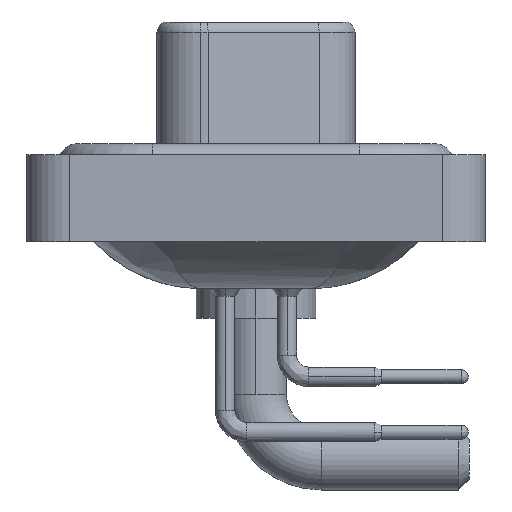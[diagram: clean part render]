
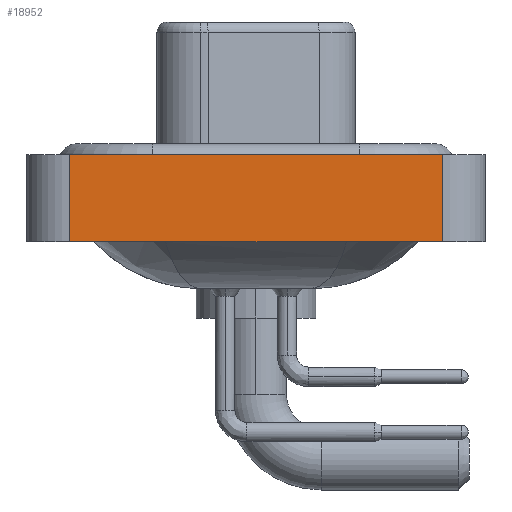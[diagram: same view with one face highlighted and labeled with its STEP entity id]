
A CAD part, left-side view. The second image highlights one B-rep face of the part: STEP entity #18952.
In plain terms, the highlighted planar face has unit normal (-1, 0, 0).
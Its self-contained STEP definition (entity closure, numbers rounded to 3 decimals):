
#564 = CARTESIAN_POINT ( 'NONE',  ( -7.25, -8.55, 0.4 ) ) ;
#1840 = AXIS2_PLACEMENT_3D ( 'NONE', #13113, #16609, #2934 ) ;
#2934 = DIRECTION ( 'NONE',  ( 0., 0., 1. ) ) ;
#3059 = ORIENTED_EDGE ( 'NONE', *, *, #8420, .T. ) ;
#3101 = EDGE_LOOP ( 'NONE', ( #10006, #10375, #14424, #3059 ) ) ;
#3458 = VERTEX_POINT ( 'NONE', #564 ) ;
#3816 = EDGE_CURVE ( 'NONE', #18432, #4788, #19182, .T. ) ;
#4437 = VECTOR ( 'NONE', #12468, 1000. ) ;
#4788 = VERTEX_POINT ( 'NONE', #21431 ) ;
#5133 = VERTEX_POINT ( 'NONE', #14258 ) ;
#5306 = EDGE_CURVE ( 'NONE', #4788, #3458, #14448, .T. ) ;
#5387 = CARTESIAN_POINT ( 'NONE',  ( -7.25, -8.55, 0.4 ) ) ;
#5415 = VECTOR ( 'NONE', #15236, 1000. ) ;
#5487 = DIRECTION ( 'NONE',  ( 0., 0., 1. ) ) ;
#7344 = CARTESIAN_POINT ( 'NONE',  ( -7.25, 8.55, -3.6 ) ) ;
#8078 = DIRECTION ( 'NONE',  ( 0., -1., 0. ) ) ;
#8420 = EDGE_CURVE ( 'NONE', #18432, #5133, #22250, .T. ) ;
#9882 = CARTESIAN_POINT ( 'NONE',  ( -7.25, -8.55, -3.6 ) ) ;
#10006 = ORIENTED_EDGE ( 'NONE', *, *, #10857, .T. ) ;
#10221 = LINE ( 'NONE', #9882, #5415 ) ;
#10375 = ORIENTED_EDGE ( 'NONE', *, *, #5306, .F. ) ;
#10857 = EDGE_CURVE ( 'NONE', #5133, #3458, #10221, .T. ) ;
#11240 = VECTOR ( 'NONE', #5487, 1000. ) ;
#12468 = DIRECTION ( 'NONE',  ( 0., -1., 0. ) ) ;
#13113 = CARTESIAN_POINT ( 'NONE',  ( -7.25, -8.55, -3.6 ) ) ;
#13234 = FACE_OUTER_BOUND ( 'NONE', #3101, .T. ) ;
#14226 = CARTESIAN_POINT ( 'NONE',  ( -7.25, 8.55, -3.6 ) ) ;
#14258 = CARTESIAN_POINT ( 'NONE',  ( -7.25, -8.55, -3.6 ) ) ;
#14424 = ORIENTED_EDGE ( 'NONE', *, *, #3816, .F. ) ;
#14448 = LINE ( 'NONE', #5387, #4437 ) ;
#15236 = DIRECTION ( 'NONE',  ( 0., 0., 1. ) ) ;
#15926 = VECTOR ( 'NONE', #8078, 1000. ) ;
#16609 = DIRECTION ( 'NONE',  ( -1., 0., 0. ) ) ;
#18432 = VERTEX_POINT ( 'NONE', #14226 ) ;
#18952 = ADVANCED_FACE ( 'NONE', ( #13234 ), #20077, .T. ) ;
#19182 = LINE ( 'NONE', #7344, #11240 ) ;
#20077 = PLANE ( 'NONE',  #1840 ) ;
#21431 = CARTESIAN_POINT ( 'NONE',  ( -7.25, 8.55, 0.4 ) ) ;
#22129 = CARTESIAN_POINT ( 'NONE',  ( -7.25, -8.55, -3.6 ) ) ;
#22250 = LINE ( 'NONE', #22129, #15926 ) ;
